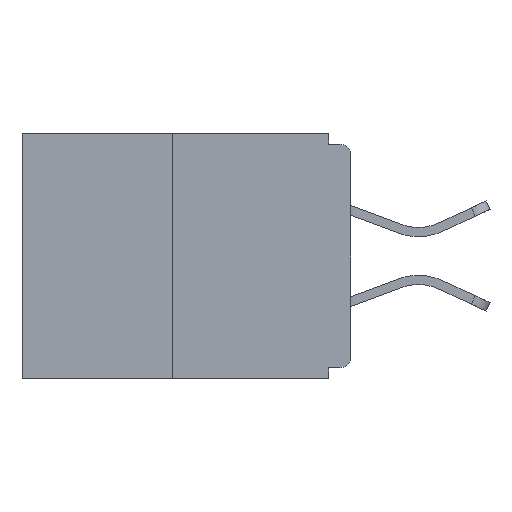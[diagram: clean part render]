
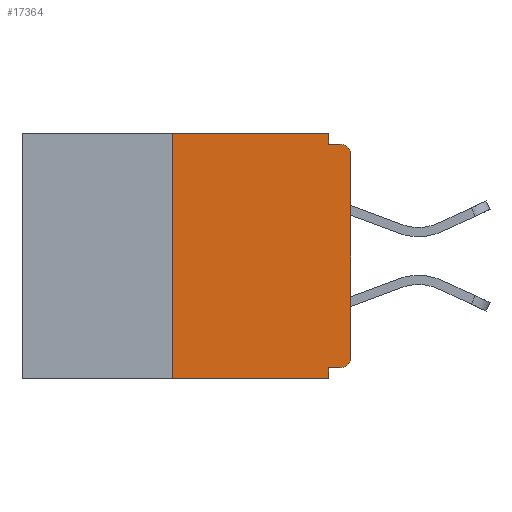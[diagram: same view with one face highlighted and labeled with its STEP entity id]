
A CAD part, left-side view. The second image highlights one B-rep face of the part: STEP entity #17364.
In plain terms, the highlighted planar face has unit normal (-1, 0, 0).
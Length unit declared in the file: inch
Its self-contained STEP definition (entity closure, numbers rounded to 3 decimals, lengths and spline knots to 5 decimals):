
#277 = VERTEX_POINT ( 'NONE', #3949 ) ;
#395 = CARTESIAN_POINT ( 'NONE',  ( 0., 0.031, -0.328 ) ) ;
#781 = CARTESIAN_POINT ( 'NONE',  ( 0., 0.25, 0. ) ) ;
#815 = AXIS2_PLACEMENT_3D ( 'NONE', #14753, #8502, #13152 ) ;
#972 = CARTESIAN_POINT ( 'NONE',  ( 0., 0.25, -0.343 ) ) ;
#1091 = DIRECTION ( 'NONE',  ( 0., -1., 0. ) ) ;
#1268 = EDGE_CURVE ( 'NONE', #16447, #8658, #14418, .T. ) ;
#1770 = VERTEX_POINT ( 'NONE', #781 ) ;
#1835 = DIRECTION ( 'NONE',  ( -1., 0., 0. ) ) ;
#2007 = DIRECTION ( 'NONE',  ( 0., -1., 0. ) ) ;
#2128 = ORIENTED_EDGE ( 'NONE', *, *, #9144, .F. ) ;
#2221 = CARTESIAN_POINT ( 'NONE',  ( 0., 0.46, 0. ) ) ;
#2328 = DIRECTION ( 'NONE',  ( 0., 0., -1. ) ) ;
#3185 = EDGE_CURVE ( 'NONE', #8550, #12092, #6749, .T. ) ;
#3470 = LINE ( 'NONE', #9990, #7536 ) ;
#3553 = DIRECTION ( 'NONE',  ( 0., 0., 1. ) ) ;
#3949 = CARTESIAN_POINT ( 'NONE',  ( 0., 0.031, -0.343 ) ) ;
#4063 = ORIENTED_EDGE ( 'NONE', *, *, #5520, .T. ) ;
#4483 = VECTOR ( 'NONE', #4661, 39.37008 ) ;
#4661 = DIRECTION ( 'NONE',  ( 0., -1., 0. ) ) ;
#5072 = CARTESIAN_POINT ( 'NONE',  ( 0., 0.46, -0.343 ) ) ;
#5347 = EDGE_LOOP ( 'NONE', ( #13178, #5623, #7364, #21112, #5873, #16710, #15604, #4063, #2128, #12664 ) ) ;
#5520 = EDGE_CURVE ( 'NONE', #12092, #18265, #7024, .T. ) ;
#5623 = ORIENTED_EDGE ( 'NONE', *, *, #7172, .F. ) ;
#5873 = ORIENTED_EDGE ( 'NONE', *, *, #1268, .F. ) ;
#5945 = FACE_OUTER_BOUND ( 'NONE', #5347, .T. ) ;
#6026 = VECTOR ( 'NONE', #3553, 39.37008 ) ;
#6149 = LINE ( 'NONE', #17328, #4483 ) ;
#6749 = LINE ( 'NONE', #18221, #6026 ) ;
#6755 = EDGE_CURVE ( 'NONE', #15132, #8460, #17806, .T. ) ;
#7024 = CIRCLE ( 'NONE', #12189, 0.015 ) ;
#7172 = EDGE_CURVE ( 'NONE', #16958, #1770, #17487, .T. ) ;
#7364 = ORIENTED_EDGE ( 'NONE', *, *, #14897, .T. ) ;
#7536 = VECTOR ( 'NONE', #16556, 39.37008 ) ;
#8412 = LINE ( 'NONE', #5072, #9576 ) ;
#8460 = VERTEX_POINT ( 'NONE', #19762 ) ;
#8502 = DIRECTION ( 'NONE',  ( -1., 0., 0. ) ) ;
#8550 = VERTEX_POINT ( 'NONE', #13142 ) ;
#8658 = VERTEX_POINT ( 'NONE', #395 ) ;
#9144 = EDGE_CURVE ( 'NONE', #8460, #18265, #14020, .T. ) ;
#9380 = VECTOR ( 'NONE', #1091, 39.37008 ) ;
#9576 = VECTOR ( 'NONE', #2007, 39.37008 ) ;
#9990 = CARTESIAN_POINT ( 'NONE',  ( 0., 0.031, -0.343 ) ) ;
#12052 = VECTOR ( 'NONE', #16031, 39.37008 ) ;
#12092 = VERTEX_POINT ( 'NONE', #18130 ) ;
#12189 = AXIS2_PLACEMENT_3D ( 'NONE', #18191, #1835, #14489 ) ;
#12664 = ORIENTED_EDGE ( 'NONE', *, *, #6755, .F. ) ;
#13118 = CARTESIAN_POINT ( 'NONE',  ( 0., 0.031, 0. ) ) ;
#13142 = CARTESIAN_POINT ( 'NONE',  ( 0., 0., -0.313 ) ) ;
#13152 = DIRECTION ( 'NONE',  ( 0., 0., -1. ) ) ;
#13178 = ORIENTED_EDGE ( 'NONE', *, *, #19233, .F. ) ;
#13333 = CARTESIAN_POINT ( 'NONE',  ( 0., 0.015, -0.015 ) ) ;
#14020 = LINE ( 'NONE', #15752, #9380 ) ;
#14418 = LINE ( 'NONE', #19429, #19440 ) ;
#14489 = DIRECTION ( 'NONE',  ( 0., 0., -1. ) ) ;
#14753 = CARTESIAN_POINT ( 'NONE',  ( 0., 0.015, -0.313 ) ) ;
#14897 = EDGE_CURVE ( 'NONE', #16958, #277, #8412, .T. ) ;
#15132 = VERTEX_POINT ( 'NONE', #13118 ) ;
#15604 = ORIENTED_EDGE ( 'NONE', *, *, #3185, .T. ) ;
#15752 = CARTESIAN_POINT ( 'NONE',  ( 0., 0., -0.015 ) ) ;
#16031 = DIRECTION ( 'NONE',  ( 0., 0., -1. ) ) ;
#16106 = DIRECTION ( 'NONE',  ( 0., 0., 1. ) ) ;
#16133 = CARTESIAN_POINT ( 'NONE',  ( 0., 0.031, 0. ) ) ;
#16447 = VERTEX_POINT ( 'NONE', #17077 ) ;
#16556 = DIRECTION ( 'NONE',  ( 0., 0., -1. ) ) ;
#16710 = ORIENTED_EDGE ( 'NONE', *, *, #17235, .T. ) ;
#16958 = VERTEX_POINT ( 'NONE', #972 ) ;
#17077 = CARTESIAN_POINT ( 'NONE',  ( 0., 0.015, -0.328 ) ) ;
#17235 = EDGE_CURVE ( 'NONE', #16447, #8550, #18559, .T. ) ;
#17328 = CARTESIAN_POINT ( 'NONE',  ( 0., 0.46, 0. ) ) ;
#17364 = ADVANCED_FACE ( 'NONE', ( #5945 ), #20520, .F. ) ;
#17487 = LINE ( 'NONE', #20824, #19295 ) ;
#17559 = AXIS2_PLACEMENT_3D ( 'NONE', #2221, #18707, #2328 ) ;
#17806 = LINE ( 'NONE', #16133, #12052 ) ;
#18130 = CARTESIAN_POINT ( 'NONE',  ( 0., 0., -0.03 ) ) ;
#18191 = CARTESIAN_POINT ( 'NONE',  ( 0., 0.015, -0.03 ) ) ;
#18221 = CARTESIAN_POINT ( 'NONE',  ( 0., 0., 0. ) ) ;
#18265 = VERTEX_POINT ( 'NONE', #13333 ) ;
#18348 = EDGE_CURVE ( 'NONE', #8658, #277, #3470, .T. ) ;
#18559 = CIRCLE ( 'NONE', #815, 0.015 ) ;
#18707 = DIRECTION ( 'NONE',  ( 1., 0., 0. ) ) ;
#19233 = EDGE_CURVE ( 'NONE', #1770, #15132, #6149, .T. ) ;
#19295 = VECTOR ( 'NONE', #16106, 39.37008 ) ;
#19429 = CARTESIAN_POINT ( 'NONE',  ( 0., 0., -0.328 ) ) ;
#19440 = VECTOR ( 'NONE', #20855, 39.37008 ) ;
#19762 = CARTESIAN_POINT ( 'NONE',  ( 0., 0.031, -0.015 ) ) ;
#20520 = PLANE ( 'NONE',  #17559 ) ;
#20824 = CARTESIAN_POINT ( 'NONE',  ( 0., 0.25, 0. ) ) ;
#20855 = DIRECTION ( 'NONE',  ( 0., 1., 0. ) ) ;
#21112 = ORIENTED_EDGE ( 'NONE', *, *, #18348, .F. ) ;
